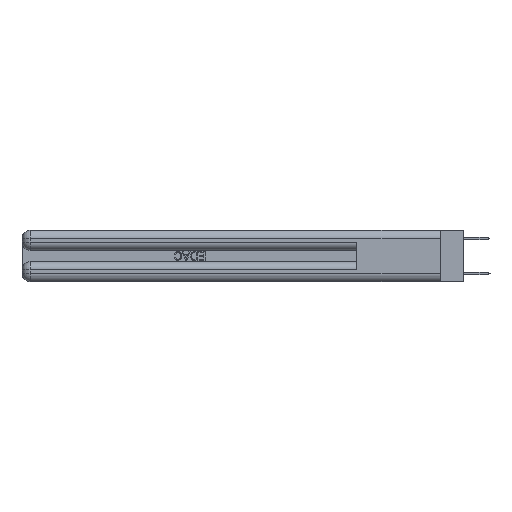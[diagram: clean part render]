
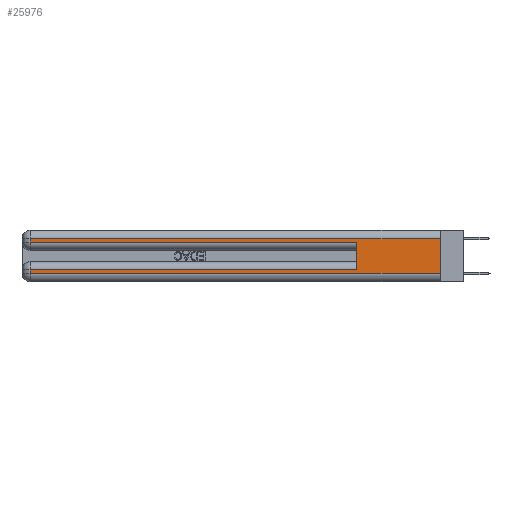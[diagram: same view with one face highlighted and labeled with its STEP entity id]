
A CAD part, left-side view. The second image highlights one B-rep face of the part: STEP entity #25976.
In plain terms, the highlighted planar face has unit normal (-1, 0, 0).
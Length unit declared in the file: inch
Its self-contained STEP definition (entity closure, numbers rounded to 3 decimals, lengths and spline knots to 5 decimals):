
#528 = ORIENTED_EDGE ( 'NONE', *, *, #18892, .T. ) ;
#1045 = EDGE_CURVE ( 'NONE', #15657, #11234, #7229, .T. ) ;
#1075 = ORIENTED_EDGE ( 'NONE', *, *, #9054, .T. ) ;
#1099 = CARTESIAN_POINT ( 'NONE',  ( 0., 2.94, 0.285 ) ) ;
#1194 = LINE ( 'NONE', #10768, #18031 ) ;
#2152 = CARTESIAN_POINT ( 'NONE',  ( 0., 0., 0.31 ) ) ;
#2271 = CARTESIAN_POINT ( 'NONE',  ( 0., 2.94, 0.31 ) ) ;
#2525 = CARTESIAN_POINT ( 'NONE',  ( 0., 0.6, 0.085 ) ) ;
#2712 = VECTOR ( 'NONE', #8117, 39.37008 ) ;
#2724 = EDGE_CURVE ( 'NONE', #23296, #11234, #18128, .T. ) ;
#2743 = EDGE_LOOP ( 'NONE', ( #4609, #24643, #528, #5005, #12575, #6123, #14909, #1075 ) ) ;
#3169 = AXIS2_PLACEMENT_3D ( 'NONE', #9258, #24422, #11447 ) ;
#3279 = DIRECTION ( 'NONE',  ( 0., 0., 1. ) ) ;
#3354 = CARTESIAN_POINT ( 'NONE',  ( 0., 0.6, 0.145 ) ) ;
#4476 = DIRECTION ( 'NONE',  ( 0., -1., 0. ) ) ;
#4609 = ORIENTED_EDGE ( 'NONE', *, *, #24944, .F. ) ;
#5005 = ORIENTED_EDGE ( 'NONE', *, *, #1045, .T. ) ;
#6123 = ORIENTED_EDGE ( 'NONE', *, *, #19412, .T. ) ;
#6608 = LINE ( 'NONE', #26983, #11736 ) ;
#7229 = LINE ( 'NONE', #14511, #7914 ) ;
#7272 = VERTEX_POINT ( 'NONE', #2152 ) ;
#7375 = VERTEX_POINT ( 'NONE', #17788 ) ;
#7904 = LINE ( 'NONE', #23230, #2712 ) ;
#7914 = VECTOR ( 'NONE', #14426, 39.37008 ) ;
#7985 = DIRECTION ( 'NONE',  ( 0., 0., -1. ) ) ;
#8117 = DIRECTION ( 'NONE',  ( 0., 1., 0. ) ) ;
#8644 = VECTOR ( 'NONE', #4476, 39.37008 ) ;
#9054 = EDGE_CURVE ( 'NONE', #15577, #17757, #14476, .T. ) ;
#9258 = CARTESIAN_POINT ( 'NONE',  ( 0., 0., 0.37 ) ) ;
#10369 = CARTESIAN_POINT ( 'NONE',  ( 0., 0., 0.06 ) ) ;
#10537 = LINE ( 'NONE', #25311, #26415 ) ;
#10768 = CARTESIAN_POINT ( 'NONE',  ( 0., 2.94, 0.37 ) ) ;
#11234 = VERTEX_POINT ( 'NONE', #23576 ) ;
#11447 = DIRECTION ( 'NONE',  ( 0., 0., -1. ) ) ;
#11634 = VECTOR ( 'NONE', #3279, 39.37008 ) ;
#11736 = VECTOR ( 'NONE', #20639, 39.37008 ) ;
#12575 = ORIENTED_EDGE ( 'NONE', *, *, #2724, .F. ) ;
#12872 = FACE_OUTER_BOUND ( 'NONE', #2743, .T. ) ;
#12979 = DIRECTION ( 'NONE',  ( 0., 0., -1. ) ) ;
#14426 = DIRECTION ( 'NONE',  ( 0., -1., 0. ) ) ;
#14476 = LINE ( 'NONE', #19769, #8644 ) ;
#14511 = CARTESIAN_POINT ( 'NONE',  ( 0., 0., 0.285 ) ) ;
#14909 = ORIENTED_EDGE ( 'NONE', *, *, #15614, .T. ) ;
#15577 = VERTEX_POINT ( 'NONE', #22635 ) ;
#15614 = EDGE_CURVE ( 'NONE', #7375, #15577, #6608, .T. ) ;
#15657 = VERTEX_POINT ( 'NONE', #1099 ) ;
#16977 = EDGE_CURVE ( 'NONE', #7272, #27043, #7904, .T. ) ;
#17157 = CARTESIAN_POINT ( 'NONE',  ( 0., 0., 0.085 ) ) ;
#17757 = VERTEX_POINT ( 'NONE', #10369 ) ;
#17788 = CARTESIAN_POINT ( 'NONE',  ( 0., 2.94, 0.085 ) ) ;
#18031 = VECTOR ( 'NONE', #12979, 39.37008 ) ;
#18128 = LINE ( 'NONE', #3354, #11634 ) ;
#18892 = EDGE_CURVE ( 'NONE', #27043, #15657, #1194, .T. ) ;
#19319 = DIRECTION ( 'NONE',  ( 0., 1., 0. ) ) ;
#19412 = EDGE_CURVE ( 'NONE', #23296, #7375, #23069, .T. ) ;
#19769 = CARTESIAN_POINT ( 'NONE',  ( 0., 0., 0.06 ) ) ;
#20639 = DIRECTION ( 'NONE',  ( 0., 0., -1. ) ) ;
#22275 = PLANE ( 'NONE',  #3169 ) ;
#22635 = CARTESIAN_POINT ( 'NONE',  ( 0., 2.94, 0.06 ) ) ;
#23069 = LINE ( 'NONE', #17157, #28022 ) ;
#23230 = CARTESIAN_POINT ( 'NONE',  ( 0., 0., 0.31 ) ) ;
#23296 = VERTEX_POINT ( 'NONE', #2525 ) ;
#23576 = CARTESIAN_POINT ( 'NONE',  ( 0., 0.6, 0.285 ) ) ;
#24422 = DIRECTION ( 'NONE',  ( 1., 0., 0. ) ) ;
#24643 = ORIENTED_EDGE ( 'NONE', *, *, #16977, .T. ) ;
#24944 = EDGE_CURVE ( 'NONE', #7272, #17757, #10537, .T. ) ;
#25311 = CARTESIAN_POINT ( 'NONE',  ( 0., 0., 0.37 ) ) ;
#25976 = ADVANCED_FACE ( 'NONE', ( #12872 ), #22275, .F. ) ;
#26415 = VECTOR ( 'NONE', #7985, 39.37008 ) ;
#26983 = CARTESIAN_POINT ( 'NONE',  ( 0., 2.94, 0.37 ) ) ;
#27043 = VERTEX_POINT ( 'NONE', #2271 ) ;
#28022 = VECTOR ( 'NONE', #19319, 39.37008 ) ;
